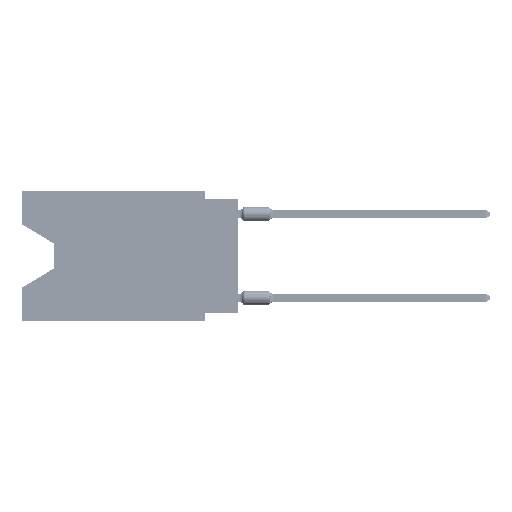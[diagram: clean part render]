
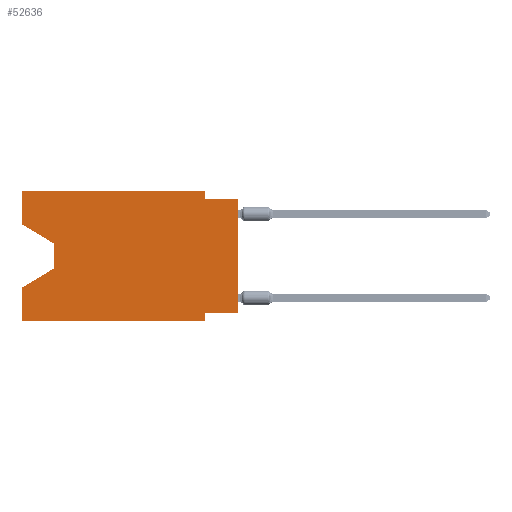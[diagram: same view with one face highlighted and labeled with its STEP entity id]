
A CAD part, left-side view. The second image highlights one B-rep face of the part: STEP entity #52636.
In plain terms, the highlighted planar face has unit normal (-1, 0, 0).
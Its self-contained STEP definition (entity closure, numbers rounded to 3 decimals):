
#2338 = DIRECTION ( 'NONE',  ( 0., 0., 1. ) ) ;
#2755 = VECTOR ( 'NONE', #14685, 1000. ) ;
#2815 = CARTESIAN_POINT ( 'NONE',  ( 0., 0., -0.635 ) ) ;
#3016 = CARTESIAN_POINT ( 'NONE',  ( 0., 13.97, -4.013 ) ) ;
#4459 = EDGE_CURVE ( 'NONE', #29707, #43317, #44156, .T. ) ;
#4743 = CARTESIAN_POINT ( 'NONE',  ( 0., 16.383, 0. ) ) ;
#5321 = ORIENTED_EDGE ( 'NONE', *, *, #17282, .F. ) ;
#6466 = LINE ( 'NONE', #6804, #34774 ) ;
#6804 = CARTESIAN_POINT ( 'NONE',  ( 0., 16.383, 0. ) ) ;
#6855 = ORIENTED_EDGE ( 'NONE', *, *, #12627, .F. ) ;
#7723 = VERTEX_POINT ( 'NONE', #43627 ) ;
#7800 = CARTESIAN_POINT ( 'NONE',  ( 0., 16.383, -9.906 ) ) ;
#11730 = DIRECTION ( 'NONE',  ( 0., 0., -1. ) ) ;
#12627 = EDGE_CURVE ( 'NONE', #53963, #43317, #18643, .T. ) ;
#13447 = CARTESIAN_POINT ( 'NONE',  ( 0., 16.383, -9.906 ) ) ;
#13466 = VERTEX_POINT ( 'NONE', #26577 ) ;
#14476 = CARTESIAN_POINT ( 'NONE',  ( 0., 0., -9.271 ) ) ;
#14685 = DIRECTION ( 'NONE',  ( 0., -1., 0. ) ) ;
#14888 = DIRECTION ( 'NONE',  ( 1., 0., 0. ) ) ;
#14899 = CARTESIAN_POINT ( 'NONE',  ( 0., 13.97, -5.893 ) ) ;
#15567 = FACE_OUTER_BOUND ( 'NONE', #65521, .T. ) ;
#15640 = CARTESIAN_POINT ( 'NONE',  ( 0., 2.54, 0. ) ) ;
#16080 = ORIENTED_EDGE ( 'NONE', *, *, #58889, .F. ) ;
#16392 = VECTOR ( 'NONE', #64794, 1000. ) ;
#17282 = EDGE_CURVE ( 'NONE', #36016, #53963, #51171, .T. ) ;
#17599 = DIRECTION ( 'NONE',  ( 0., -1., 0. ) ) ;
#18466 = VECTOR ( 'NONE', #29836, 1000. ) ;
#18643 = LINE ( 'NONE', #50798, #40215 ) ;
#18804 = CARTESIAN_POINT ( 'NONE',  ( 0., 0., -9.271 ) ) ;
#18960 = ORIENTED_EDGE ( 'NONE', *, *, #45153, .T. ) ;
#19075 = LINE ( 'NONE', #45287, #68263 ) ;
#19140 = CARTESIAN_POINT ( 'NONE',  ( 0., 16.383, 0. ) ) ;
#19273 = LINE ( 'NONE', #49116, #26139 ) ;
#19435 = LINE ( 'NONE', #14899, #58155 ) ;
#20031 = CARTESIAN_POINT ( 'NONE',  ( 0., 13.97, -5.893 ) ) ;
#21367 = EDGE_CURVE ( 'NONE', #36016, #68832, #34132, .T. ) ;
#23798 = ORIENTED_EDGE ( 'NONE', *, *, #40162, .F. ) ;
#25427 = VERTEX_POINT ( 'NONE', #43508 ) ;
#26139 = VECTOR ( 'NONE', #11730, 1000. ) ;
#26577 = CARTESIAN_POINT ( 'NONE',  ( 0., 2.54, -0.635 ) ) ;
#27344 = VERTEX_POINT ( 'NONE', #37077 ) ;
#28860 = EDGE_CURVE ( 'NONE', #29707, #25427, #47829, .T. ) ;
#29440 = ORIENTED_EDGE ( 'NONE', *, *, #4459, .T. ) ;
#29707 = VERTEX_POINT ( 'NONE', #13447 ) ;
#29836 = DIRECTION ( 'NONE',  ( 0., 1., 0. ) ) ;
#31659 = EDGE_CURVE ( 'NONE', #13466, #68832, #32878, .T. ) ;
#31696 = DIRECTION ( 'NONE',  ( 0., 0., -1. ) ) ;
#32313 = LINE ( 'NONE', #53640, #16392 ) ;
#32878 = LINE ( 'NONE', #2815, #2755 ) ;
#33851 = ORIENTED_EDGE ( 'NONE', *, *, #31659, .F. ) ;
#34132 = LINE ( 'NONE', #50217, #56841 ) ;
#34774 = VECTOR ( 'NONE', #60247, 1000. ) ;
#35832 = DIRECTION ( 'NONE',  ( 0., 0., -1. ) ) ;
#36016 = VERTEX_POINT ( 'NONE', #18804 ) ;
#36930 = ORIENTED_EDGE ( 'NONE', *, *, #21367, .T. ) ;
#37016 = VERTEX_POINT ( 'NONE', #19140 ) ;
#37077 = CARTESIAN_POINT ( 'NONE',  ( 0., 16.383, -2.546 ) ) ;
#38308 = ORIENTED_EDGE ( 'NONE', *, *, #44551, .T. ) ;
#38654 = VERTEX_POINT ( 'NONE', #3016 ) ;
#40162 = EDGE_CURVE ( 'NONE', #27344, #37016, #6466, .T. ) ;
#40215 = VECTOR ( 'NONE', #56033, 1000. ) ;
#40754 = DIRECTION ( 'NONE',  ( 0., 0.855, -0.519 ) ) ;
#42928 = AXIS2_PLACEMENT_3D ( 'NONE', #4743, #14888, #35832 ) ;
#43317 = VERTEX_POINT ( 'NONE', #47962 ) ;
#43508 = CARTESIAN_POINT ( 'NONE',  ( 0., 16.383, -7.36 ) ) ;
#43627 = CARTESIAN_POINT ( 'NONE',  ( 0., 2.54, 0. ) ) ;
#44133 = VECTOR ( 'NONE', #31696, 1000. ) ;
#44156 = LINE ( 'NONE', #7800, #55124 ) ;
#44235 = ORIENTED_EDGE ( 'NONE', *, *, #48993, .F. ) ;
#44551 = EDGE_CURVE ( 'NONE', #45411, #25427, #19435, .T. ) ;
#45153 = EDGE_CURVE ( 'NONE', #27344, #38654, #32313, .T. ) ;
#45287 = CARTESIAN_POINT ( 'NONE',  ( 0., 16.383, 0. ) ) ;
#45411 = VERTEX_POINT ( 'NONE', #20031 ) ;
#47829 = LINE ( 'NONE', #48860, #53806 ) ;
#47962 = CARTESIAN_POINT ( 'NONE',  ( 0., 2.54, -9.906 ) ) ;
#48860 = CARTESIAN_POINT ( 'NONE',  ( 0., 16.383, 0. ) ) ;
#48993 = EDGE_CURVE ( 'NONE', #37016, #7723, #19075, .T. ) ;
#49116 = CARTESIAN_POINT ( 'NONE',  ( 0., 13.97, -4.013 ) ) ;
#50217 = CARTESIAN_POINT ( 'NONE',  ( 0., 0., 0. ) ) ;
#50798 = CARTESIAN_POINT ( 'NONE',  ( 0., 2.54, -9.906 ) ) ;
#51171 = LINE ( 'NONE', #14476, #18466 ) ;
#52636 = ADVANCED_FACE ( 'NONE', ( #15567 ), #62382, .F. ) ;
#53640 = CARTESIAN_POINT ( 'NONE',  ( 0., 16.383, -2.546 ) ) ;
#53806 = VECTOR ( 'NONE', #59678, 1000. ) ;
#53963 = VERTEX_POINT ( 'NONE', #62742 ) ;
#55124 = VECTOR ( 'NONE', #17599, 1000. ) ;
#55554 = EDGE_CURVE ( 'NONE', #38654, #45411, #19273, .T. ) ;
#56033 = DIRECTION ( 'NONE',  ( 0., 0., -1. ) ) ;
#56467 = ORIENTED_EDGE ( 'NONE', *, *, #28860, .F. ) ;
#56841 = VECTOR ( 'NONE', #2338, 1000. ) ;
#58155 = VECTOR ( 'NONE', #40754, 1000. ) ;
#58169 = ORIENTED_EDGE ( 'NONE', *, *, #55554, .T. ) ;
#58889 = EDGE_CURVE ( 'NONE', #7723, #13466, #63836, .T. ) ;
#59678 = DIRECTION ( 'NONE',  ( 0., 0., 1. ) ) ;
#60247 = DIRECTION ( 'NONE',  ( 0., 0., 1. ) ) ;
#62382 = PLANE ( 'NONE',  #42928 ) ;
#62742 = CARTESIAN_POINT ( 'NONE',  ( 0., 2.54, -9.271 ) ) ;
#63836 = LINE ( 'NONE', #15640, #44133 ) ;
#64794 = DIRECTION ( 'NONE',  ( 0., -0.855, -0.519 ) ) ;
#65521 = EDGE_LOOP ( 'NONE', ( #18960, #58169, #38308, #56467, #29440, #6855, #5321, #36930, #33851, #16080, #44235, #23798 ) ) ;
#66256 = DIRECTION ( 'NONE',  ( 0., -1., 0. ) ) ;
#66307 = CARTESIAN_POINT ( 'NONE',  ( 0., 0., -0.635 ) ) ;
#68263 = VECTOR ( 'NONE', #66256, 1000. ) ;
#68832 = VERTEX_POINT ( 'NONE', #66307 ) ;
